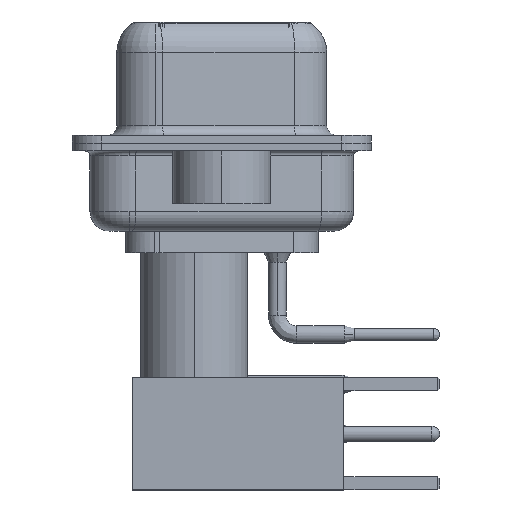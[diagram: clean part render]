
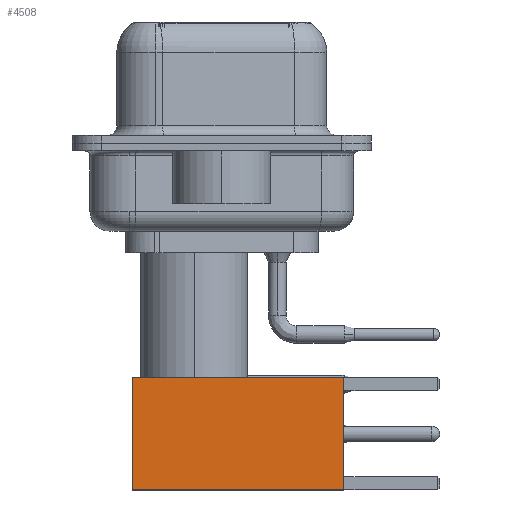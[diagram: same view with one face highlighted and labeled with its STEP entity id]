
A CAD part, left-side view. The second image highlights one B-rep face of the part: STEP entity #4508.
In plain terms, the highlighted face is planar.
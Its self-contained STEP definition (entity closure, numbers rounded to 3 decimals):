
#2133 = VERTEX_POINT ( 'NONE', #27584 ) ;
#2822 = LINE ( 'NONE', #28223, #9421 ) ;
#3112 = DIRECTION ( 'NONE',  ( 0., 1., 0. ) ) ;
#3568 = ORIENTED_EDGE ( 'NONE', *, *, #25790, .F. ) ;
#4508 = ADVANCED_FACE ( 'NONE', ( #16060 ), #26664, .T. ) ;
#4579 = CARTESIAN_POINT ( 'NONE',  ( 2.875, 2.875, 0. ) ) ;
#5812 = VECTOR ( 'NONE', #18214, 1000. ) ;
#6279 = DIRECTION ( 'NONE',  ( 0., 0., 1. ) ) ;
#8715 = VECTOR ( 'NONE', #32577, 1000. ) ;
#9313 = CARTESIAN_POINT ( 'NONE',  ( 0., 2.875, 0. ) ) ;
#9421 = VECTOR ( 'NONE', #18277, 1000. ) ;
#10616 = CARTESIAN_POINT ( 'NONE',  ( 0., 2.875, 10.82 ) ) ;
#11310 = ORIENTED_EDGE ( 'NONE', *, *, #12241, .F. ) ;
#12241 = EDGE_CURVE ( 'NONE', #2133, #26074, #26118, .T. ) ;
#12310 = DIRECTION ( 'NONE',  ( 0., 0., -1. ) ) ;
#13140 = AXIS2_PLACEMENT_3D ( 'NONE', #18748, #3112, #6279 ) ;
#13196 = VERTEX_POINT ( 'NONE', #18307 ) ;
#16060 = FACE_OUTER_BOUND ( 'NONE', #24339, .T. ) ;
#17381 = EDGE_CURVE ( 'NONE', #13196, #19820, #26687, .T. ) ;
#18214 = DIRECTION ( 'NONE',  ( -1., 0., 0. ) ) ;
#18277 = DIRECTION ( 'NONE',  ( 0., 0., -1. ) ) ;
#18307 = CARTESIAN_POINT ( 'NONE',  ( 2.875, 2.875, 0. ) ) ;
#18748 = CARTESIAN_POINT ( 'NONE',  ( 2.875, 2.875, 0. ) ) ;
#19820 = VERTEX_POINT ( 'NONE', #30299 ) ;
#24339 = EDGE_LOOP ( 'NONE', ( #32992, #28709, #3568, #11310 ) ) ;
#25290 = EDGE_CURVE ( 'NONE', #2133, #13196, #29986, .T. ) ;
#25790 = EDGE_CURVE ( 'NONE', #26074, #19820, #2822, .T. ) ;
#26074 = VERTEX_POINT ( 'NONE', #29218 ) ;
#26118 = LINE ( 'NONE', #10616, #5812 ) ;
#26664 = PLANE ( 'NONE',  #13140 ) ;
#26687 = LINE ( 'NONE', #9313, #8715 ) ;
#27584 = CARTESIAN_POINT ( 'NONE',  ( 2.875, 2.875, 10.82 ) ) ;
#28223 = CARTESIAN_POINT ( 'NONE',  ( -2.875, 2.875, 0. ) ) ;
#28709 = ORIENTED_EDGE ( 'NONE', *, *, #17381, .T. ) ;
#29218 = CARTESIAN_POINT ( 'NONE',  ( -2.875, 2.875, 10.82 ) ) ;
#29986 = LINE ( 'NONE', #4579, #32093 ) ;
#30299 = CARTESIAN_POINT ( 'NONE',  ( -2.875, 2.875, 0. ) ) ;
#32093 = VECTOR ( 'NONE', #12310, 1000. ) ;
#32577 = DIRECTION ( 'NONE',  ( -1., 0., 0. ) ) ;
#32992 = ORIENTED_EDGE ( 'NONE', *, *, #25290, .T. ) ;
